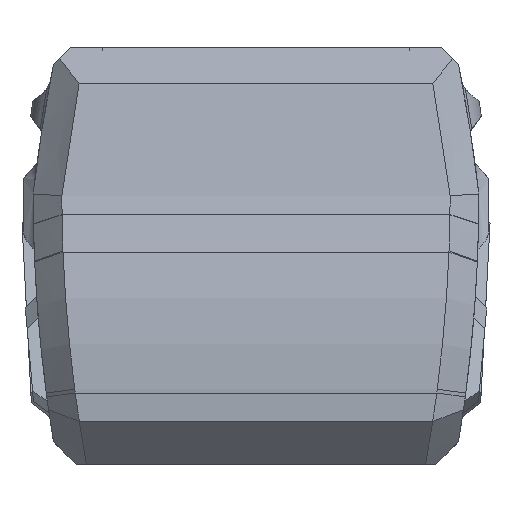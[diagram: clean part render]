
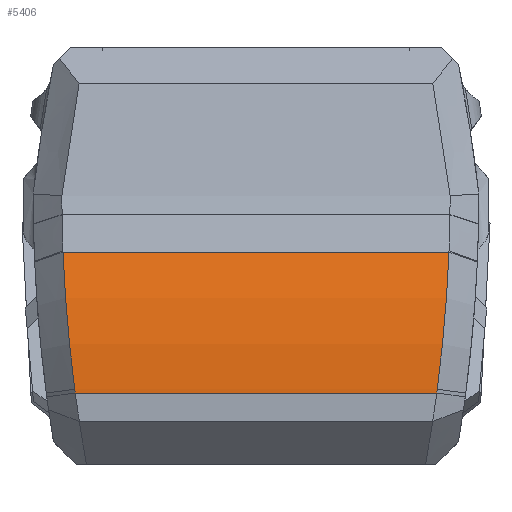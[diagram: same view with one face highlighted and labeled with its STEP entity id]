
A CAD part, front view. The second image highlights one B-rep face of the part: STEP entity #5406.
In plain terms, the highlighted cylindrical face has radius 31 mm (diameter 62 mm), a partial arc.
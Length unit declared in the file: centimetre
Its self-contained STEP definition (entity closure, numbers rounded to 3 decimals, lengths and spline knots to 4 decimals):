
#137=B_SPLINE_CURVE_WITH_KNOTS($,3,(#9229,#9230,#9231,#9232),
 .UNSPECIFIED.,.F.,.F.,(4,4),(-4.6815,-3.7231),
 .UNSPECIFIED.);
#138=B_SPLINE_CURVE_WITH_KNOTS($,3,(#9249,#9250,#9251,#9252),
 .UNSPECIFIED.,.F.,.F.,(4,4),(0.0299,0.0324),
 .UNSPECIFIED.);
#149=B_SPLINE_CURVE_WITH_KNOTS($,3,(#9437,#9438,#9439,#9440),
 .UNSPECIFIED.,.F.,.F.,(4,4),(-5.7254,-4.767),
 .UNSPECIFIED.);
#158=B_SPLINE_CURVE_WITH_KNOTS($,3,(#9585,#9586,#9587,#9588),
 .UNSPECIFIED.,.F.,.F.,(4,4),(-0.0324,-0.0299),
 .UNSPECIFIED.);
#376=CYLINDRICAL_SURFACE($,#5821,3.1);
#634=FACE_OUTER_BOUND($,#945,.T.);
#945=EDGE_LOOP($,(#4768,#4769,#4770,#4771,#4772,#4773));
#1464=LINE($,#9590,#1992);
#1465=LINE($,#9592,#1993);
#1992=VECTOR($,#7102,2.5143);
#1993=VECTOR($,#7105,2.6843);
#2520=VERTEX_POINT($,#9175);
#2522=VERTEX_POINT($,#9225);
#2523=VERTEX_POINT($,#9227);
#2532=VERTEX_POINT($,#9415);
#2533=VERTEX_POINT($,#9434);
#2534=VERTEX_POINT($,#9436);
#3270=EDGE_CURVE($,#2523,#2522,#137,.T.);
#3271=EDGE_CURVE($,#2520,#2523,#138,.T.);
#3290=EDGE_CURVE($,#2533,#2534,#149,.T.);
#3303=EDGE_CURVE($,#2534,#2532,#158,.T.);
#3304=EDGE_CURVE($,#2520,#2532,#1464,.T.);
#3305=EDGE_CURVE($,#2533,#2522,#1465,.T.);
#4768=ORIENTED_EDGE($,*,*,#3271,.F.);
#4769=ORIENTED_EDGE($,*,*,#3304,.T.);
#4770=ORIENTED_EDGE($,*,*,#3303,.F.);
#4771=ORIENTED_EDGE($,*,*,#3290,.F.);
#4772=ORIENTED_EDGE($,*,*,#3305,.T.);
#4773=ORIENTED_EDGE($,*,*,#3270,.F.);
#5406=ADVANCED_FACE($,(#634),#376,.T.);
#5821=AXIS2_PLACEMENT_3D($,#9591,#7103,#7104);
#7102=DIRECTION($,(1.,0.,0.));
#7103=DIRECTION('center_axis',(-1.,0.,0.));
#7104=DIRECTION('ref_axis',(0.,-0.987,0.16));
#7105=DIRECTION($,(-1.,0.,0.));
#9175=CARTESIAN_POINT('',(-9.7046,11.8345,15.2164));
#9225=CARTESIAN_POINT('',(-9.7896,11.9936,16.1967));
#9227=CARTESIAN_POINT('',(-9.7081,11.8346,15.2426));
#9229=CARTESIAN_POINT('Ctrl Pts',(-9.7081,11.8346,15.2426));
#9230=CARTESIAN_POINT('Ctrl Pts',(-9.7492,11.8373,15.5533));
#9231=CARTESIAN_POINT('Ctrl Pts',(-9.7774,11.8886,15.8818));
#9232=CARTESIAN_POINT('Ctrl Pts',(-9.7896,11.9936,16.1967));
#9249=CARTESIAN_POINT('Ctrl Pts',(-9.7046,11.8345,15.2164));
#9250=CARTESIAN_POINT('Ctrl Pts',(-9.7058,11.8345,15.2251));
#9251=CARTESIAN_POINT('Ctrl Pts',(-9.707,11.8346,15.2339));
#9252=CARTESIAN_POINT('Ctrl Pts',(-9.7081,11.8346,15.2426));
#9415=CARTESIAN_POINT('',(-7.1903,11.8345,15.2164));
#9434=CARTESIAN_POINT('',(-7.1053,11.9936,16.1967));
#9436=CARTESIAN_POINT('',(-7.1868,11.8346,15.2426));
#9437=CARTESIAN_POINT('Ctrl Pts',(-7.1053,11.9936,16.1967));
#9438=CARTESIAN_POINT('Ctrl Pts',(-7.1176,11.8886,15.8818));
#9439=CARTESIAN_POINT('Ctrl Pts',(-7.1457,11.8373,15.5533));
#9440=CARTESIAN_POINT('Ctrl Pts',(-7.1868,11.8346,15.2426));
#9585=CARTESIAN_POINT('Ctrl Pts',(-7.1868,11.8346,15.2426));
#9586=CARTESIAN_POINT('Ctrl Pts',(-7.188,11.8346,15.2339));
#9587=CARTESIAN_POINT('Ctrl Pts',(-7.1892,11.8345,15.2251));
#9588=CARTESIAN_POINT('Ctrl Pts',(-7.1903,11.8345,15.2164));
#9590=CARTESIAN_POINT($,(-9.8475,11.8345,15.2164));
#9591=CARTESIAN_POINT('Origin',(-9.8475,14.9345,15.2164));
#9592=CARTESIAN_POINT($,(-9.8475,11.9936,16.1967));
